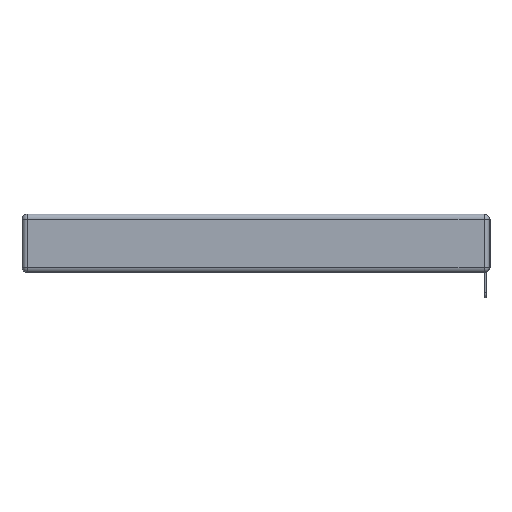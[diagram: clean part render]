
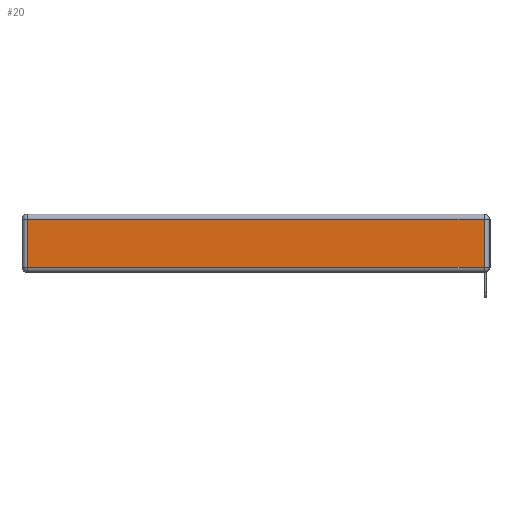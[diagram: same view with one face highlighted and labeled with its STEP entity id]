
A CAD part, left-side view. The second image highlights one B-rep face of the part: STEP entity #20.
In plain terms, the highlighted planar face has unit normal (-1, 0, 0).
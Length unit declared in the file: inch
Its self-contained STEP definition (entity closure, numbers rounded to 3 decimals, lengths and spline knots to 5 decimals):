
#20 = ADVANCED_FACE ( 'NONE', ( #10662 ), #7035, .T. ) ;
#882 = DIRECTION ( 'NONE',  ( -1., 0., 0. ) ) ;
#1196 = CARTESIAN_POINT ( 'NONE',  ( 0., 2.72, -0.313 ) ) ;
#1280 = ORIENTED_EDGE ( 'NONE', *, *, #2995, .T. ) ;
#1976 = DIRECTION ( 'NONE',  ( 0., -1., 0. ) ) ;
#2392 = VECTOR ( 'NONE', #8272, 39.37008 ) ;
#2652 = CARTESIAN_POINT ( 'NONE',  ( 0., 0.03, -0.343 ) ) ;
#2797 = DIRECTION ( 'NONE',  ( 0., 0., 1. ) ) ;
#2977 = DIRECTION ( 'NONE',  ( 0., 1., 0. ) ) ;
#2995 = EDGE_CURVE ( 'NONE', #12835, #7424, #5388, .T. ) ;
#3063 = ORIENTED_EDGE ( 'NONE', *, *, #7604, .T. ) ;
#3278 = VECTOR ( 'NONE', #2977, 39.37008 ) ;
#3800 = LINE ( 'NONE', #10138, #4950 ) ;
#4243 = CARTESIAN_POINT ( 'NONE',  ( 0., 0.03, -0.03 ) ) ;
#4950 = VECTOR ( 'NONE', #1976, 39.37008 ) ;
#5070 = LINE ( 'NONE', #10382, #12486 ) ;
#5388 = LINE ( 'NONE', #10187, #3278 ) ;
#5947 = CARTESIAN_POINT ( 'NONE',  ( 0., 0., -0.343 ) ) ;
#6305 = DIRECTION ( 'NONE',  ( 0., 0., -1. ) ) ;
#6731 = VERTEX_POINT ( 'NONE', #1196 ) ;
#6739 = ORIENTED_EDGE ( 'NONE', *, *, #12134, .T. ) ;
#6870 = AXIS2_PLACEMENT_3D ( 'NONE', #5947, #882, #2797 ) ;
#7035 = PLANE ( 'NONE',  #6870 ) ;
#7424 = VERTEX_POINT ( 'NONE', #12877 ) ;
#7604 = EDGE_CURVE ( 'NONE', #6731, #11850, #3800, .T. ) ;
#8272 = DIRECTION ( 'NONE',  ( 0., 0., 1. ) ) ;
#8399 = CARTESIAN_POINT ( 'NONE',  ( 0., 0.03, -0.313 ) ) ;
#9017 = EDGE_CURVE ( 'NONE', #7424, #6731, #5070, .T. ) ;
#9687 = ORIENTED_EDGE ( 'NONE', *, *, #9017, .T. ) ;
#9816 = LINE ( 'NONE', #2652, #2392 ) ;
#10138 = CARTESIAN_POINT ( 'NONE',  ( 0., 0., -0.313 ) ) ;
#10187 = CARTESIAN_POINT ( 'NONE',  ( 0., 2.75, -0.03 ) ) ;
#10382 = CARTESIAN_POINT ( 'NONE',  ( 0., 2.72, -0.343 ) ) ;
#10662 = FACE_OUTER_BOUND ( 'NONE', #11639, .T. ) ;
#11639 = EDGE_LOOP ( 'NONE', ( #3063, #6739, #1280, #9687 ) ) ;
#11850 = VERTEX_POINT ( 'NONE', #8399 ) ;
#12134 = EDGE_CURVE ( 'NONE', #11850, #12835, #9816, .T. ) ;
#12486 = VECTOR ( 'NONE', #6305, 39.37008 ) ;
#12835 = VERTEX_POINT ( 'NONE', #4243 ) ;
#12877 = CARTESIAN_POINT ( 'NONE',  ( 0., 2.72, -0.03 ) ) ;
